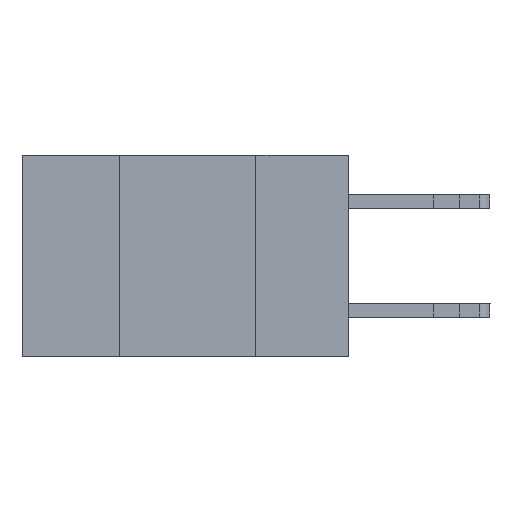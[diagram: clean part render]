
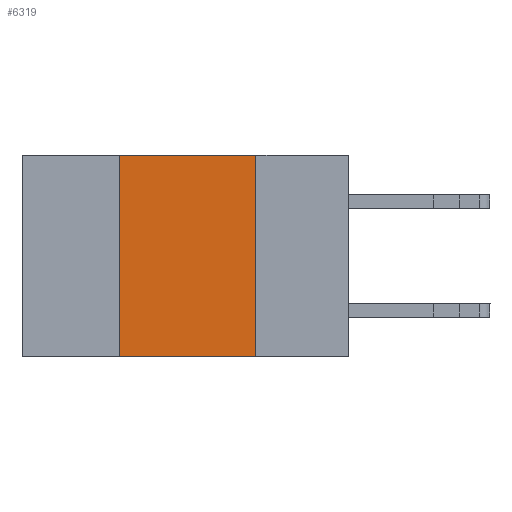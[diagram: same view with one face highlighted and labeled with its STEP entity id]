
A CAD part, left-side view. The second image highlights one B-rep face of the part: STEP entity #6319.
In plain terms, the highlighted planar face has unit normal (-1, 0, 0).
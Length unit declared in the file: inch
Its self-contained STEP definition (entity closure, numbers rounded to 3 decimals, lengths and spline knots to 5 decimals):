
#57 = EDGE_LOOP ( 'NONE', ( #16321, #7258, #23436, #16629 ) ) ;
#112 = AXIS2_PLACEMENT_3D ( 'NONE', #17847, #9727, #7263 ) ;
#846 = DIRECTION ( 'NONE',  ( 0., 0., -1. ) ) ;
#1157 = EDGE_CURVE ( 'NONE', #5138, #24812, #26313, .T. ) ;
#1172 = DIRECTION ( 'NONE',  ( 0., 0., 1. ) ) ;
#2554 = VECTOR ( 'NONE', #27438, 39.37008 ) ;
#4008 = CARTESIAN_POINT ( 'NONE',  ( 0., 0.42, -0.37 ) ) ;
#5138 = VERTEX_POINT ( 'NONE', #4008 ) ;
#6319 = ADVANCED_FACE ( 'NONE', ( #20764 ), #11793, .F. ) ;
#6831 = VECTOR ( 'NONE', #24323, 39.37008 ) ;
#7124 = EDGE_CURVE ( 'NONE', #24812, #25025, #24657, .T. ) ;
#7258 = ORIENTED_EDGE ( 'NONE', *, *, #7124, .F. ) ;
#7263 = DIRECTION ( 'NONE',  ( 0., 0., -1. ) ) ;
#8813 = EDGE_CURVE ( 'NONE', #25025, #17567, #25958, .T. ) ;
#9664 = CARTESIAN_POINT ( 'NONE',  ( 0., 0.42, 0. ) ) ;
#9727 = DIRECTION ( 'NONE',  ( 1., 0., 0. ) ) ;
#11793 = PLANE ( 'NONE',  #112 ) ;
#12029 = CARTESIAN_POINT ( 'NONE',  ( 0., 0.42, 0. ) ) ;
#13175 = EDGE_CURVE ( 'NONE', #5138, #17567, #13191, .T. ) ;
#13191 = LINE ( 'NONE', #25312, #2554 ) ;
#13487 = CARTESIAN_POINT ( 'NONE',  ( 0., 0.17, 0. ) ) ;
#16321 = ORIENTED_EDGE ( 'NONE', *, *, #8813, .F. ) ;
#16513 = CARTESIAN_POINT ( 'NONE',  ( 0., 0.17, 0. ) ) ;
#16629 = ORIENTED_EDGE ( 'NONE', *, *, #13175, .T. ) ;
#17567 = VERTEX_POINT ( 'NONE', #27176 ) ;
#17847 = CARTESIAN_POINT ( 'NONE',  ( 0., 0.6, 0. ) ) ;
#20708 = VECTOR ( 'NONE', #1172, 39.37008 ) ;
#20764 = FACE_OUTER_BOUND ( 'NONE', #57, .T. ) ;
#22208 = CARTESIAN_POINT ( 'NONE',  ( 0., 0.6, 0. ) ) ;
#22300 = VECTOR ( 'NONE', #846, 39.37008 ) ;
#23436 = ORIENTED_EDGE ( 'NONE', *, *, #1157, .F. ) ;
#24323 = DIRECTION ( 'NONE',  ( 0., -1., 0. ) ) ;
#24657 = LINE ( 'NONE', #22208, #6831 ) ;
#24812 = VERTEX_POINT ( 'NONE', #12029 ) ;
#25025 = VERTEX_POINT ( 'NONE', #16513 ) ;
#25312 = CARTESIAN_POINT ( 'NONE',  ( 0., 0.6, -0.37 ) ) ;
#25958 = LINE ( 'NONE', #13487, #22300 ) ;
#26313 = LINE ( 'NONE', #9664, #20708 ) ;
#27176 = CARTESIAN_POINT ( 'NONE',  ( 0., 0.17, -0.37 ) ) ;
#27438 = DIRECTION ( 'NONE',  ( 0., -1., 0. ) ) ;
